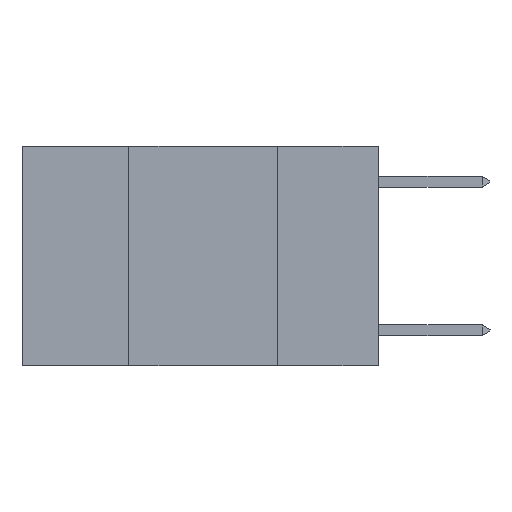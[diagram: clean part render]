
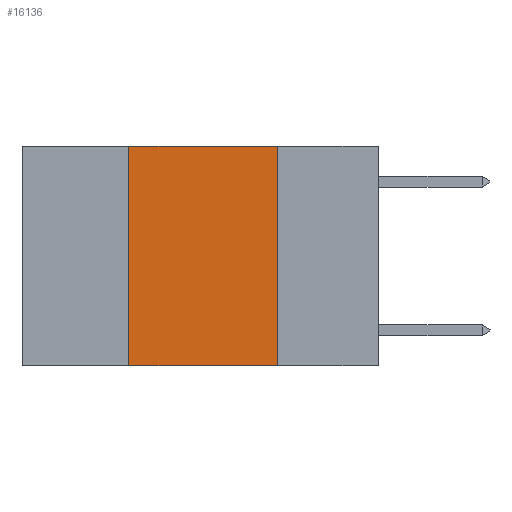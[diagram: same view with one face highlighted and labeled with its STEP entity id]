
A CAD part, left-side view. The second image highlights one B-rep face of the part: STEP entity #16136.
In plain terms, the highlighted planar face has unit normal (-1, 0, 0).
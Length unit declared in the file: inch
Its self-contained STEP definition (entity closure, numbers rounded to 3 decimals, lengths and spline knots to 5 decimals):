
#37 = CARTESIAN_POINT ( 'NONE',  ( 0., 0.42, -0.37 ) ) ;
#612 = ORIENTED_EDGE ( 'NONE', *, *, #7737, .T. ) ;
#645 = EDGE_CURVE ( 'NONE', #20424, #4076, #9418, .T. ) ;
#676 = DIRECTION ( 'NONE',  ( 0., -1., 0. ) ) ;
#820 = CARTESIAN_POINT ( 'NONE',  ( 0., 0.6, -0.37 ) ) ;
#1178 = FACE_OUTER_BOUND ( 'NONE', #20358, .T. ) ;
#2508 = ORIENTED_EDGE ( 'NONE', *, *, #645, .F. ) ;
#4076 = VERTEX_POINT ( 'NONE', #16432 ) ;
#4797 = VECTOR ( 'NONE', #15250, 39.37008 ) ;
#4823 = LINE ( 'NONE', #15455, #4797 ) ;
#5814 = VERTEX_POINT ( 'NONE', #7841 ) ;
#6280 = DIRECTION ( 'NONE',  ( 0., 0., -1. ) ) ;
#6350 = DIRECTION ( 'NONE',  ( 1., 0., 0. ) ) ;
#6376 = PLANE ( 'NONE',  #17092 ) ;
#6434 = DIRECTION ( 'NONE',  ( 0., -1., 0. ) ) ;
#6498 = VERTEX_POINT ( 'NONE', #37 ) ;
#6712 = CARTESIAN_POINT ( 'NONE',  ( 0., 0.6, 0. ) ) ;
#7737 = EDGE_CURVE ( 'NONE', #6498, #5814, #10606, .T. ) ;
#7841 = CARTESIAN_POINT ( 'NONE',  ( 0., 0.17, -0.37 ) ) ;
#8813 = EDGE_CURVE ( 'NONE', #6498, #20424, #4823, .T. ) ;
#9418 = LINE ( 'NONE', #16902, #9519 ) ;
#9519 = VECTOR ( 'NONE', #6434, 39.37008 ) ;
#10429 = VECTOR ( 'NONE', #676, 39.37008 ) ;
#10606 = LINE ( 'NONE', #820, #10429 ) ;
#11001 = EDGE_CURVE ( 'NONE', #4076, #5814, #14072, .T. ) ;
#11456 = DIRECTION ( 'NONE',  ( 0., 0., -1. ) ) ;
#12036 = CARTESIAN_POINT ( 'NONE',  ( 0., 0.17, 0. ) ) ;
#13061 = ORIENTED_EDGE ( 'NONE', *, *, #8813, .F. ) ;
#14011 = ORIENTED_EDGE ( 'NONE', *, *, #11001, .F. ) ;
#14034 = VECTOR ( 'NONE', #11456, 39.37008 ) ;
#14072 = LINE ( 'NONE', #12036, #14034 ) ;
#15250 = DIRECTION ( 'NONE',  ( 0., 0., 1. ) ) ;
#15455 = CARTESIAN_POINT ( 'NONE',  ( 0., 0.42, 0. ) ) ;
#16136 = ADVANCED_FACE ( 'NONE', ( #1178 ), #6376, .F. ) ;
#16432 = CARTESIAN_POINT ( 'NONE',  ( 0., 0.17, 0. ) ) ;
#16902 = CARTESIAN_POINT ( 'NONE',  ( 0., 0.6, 0. ) ) ;
#17092 = AXIS2_PLACEMENT_3D ( 'NONE', #6712, #6350, #6280 ) ;
#18274 = CARTESIAN_POINT ( 'NONE',  ( 0., 0.42, 0. ) ) ;
#20358 = EDGE_LOOP ( 'NONE', ( #14011, #2508, #13061, #612 ) ) ;
#20424 = VERTEX_POINT ( 'NONE', #18274 ) ;
